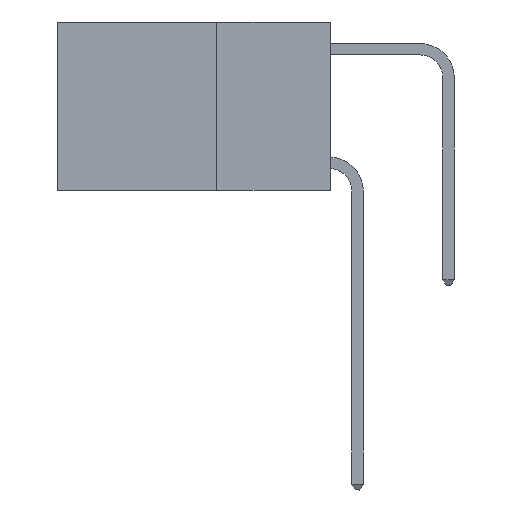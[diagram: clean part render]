
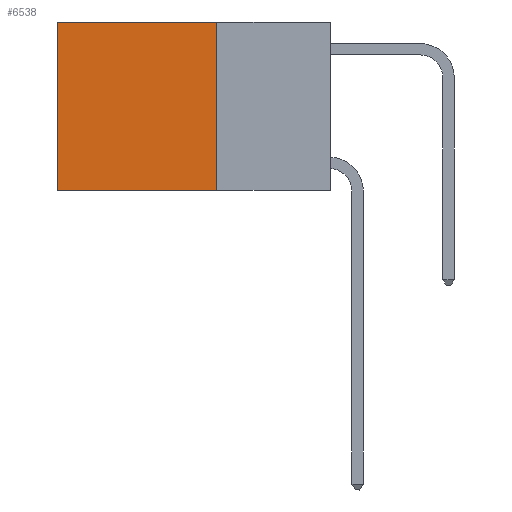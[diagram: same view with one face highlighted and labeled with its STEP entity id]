
A CAD part, left-side view. The second image highlights one B-rep face of the part: STEP entity #6538.
In plain terms, the highlighted planar face has unit normal (-1, 0, 0).
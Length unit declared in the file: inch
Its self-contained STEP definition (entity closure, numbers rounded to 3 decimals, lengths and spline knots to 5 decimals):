
#830 = PLANE ( 'NONE',  #6631 ) ;
#2566 = EDGE_CURVE ( 'NONE', #31942, #11204, #31097, .T. ) ;
#3371 = DIRECTION ( 'NONE',  ( 0., 0., -1. ) ) ;
#3516 = FACE_OUTER_BOUND ( 'NONE', #16178, .T. ) ;
#3772 = ORIENTED_EDGE ( 'NONE', *, *, #16917, .F. ) ;
#5088 = VECTOR ( 'NONE', #30983, 39.37008 ) ;
#5108 = CARTESIAN_POINT ( 'NONE',  ( 0.2625, 0.25, -0.37 ) ) ;
#5208 = CARTESIAN_POINT ( 'NONE',  ( 0.2625, 0.6, 0. ) ) ;
#5916 = LINE ( 'NONE', #5108, #5088 ) ;
#6202 = LINE ( 'NONE', #27113, #25265 ) ;
#6538 = ADVANCED_FACE ( 'NONE', ( #3516 ), #830, .F. ) ;
#6631 = AXIS2_PLACEMENT_3D ( 'NONE', #16211, #18812, #3371 ) ;
#7097 = CARTESIAN_POINT ( 'NONE',  ( 0.2625, 0.6, 0. ) ) ;
#8294 = EDGE_CURVE ( 'NONE', #31942, #12168, #6202, .T. ) ;
#8778 = CARTESIAN_POINT ( 'NONE',  ( 0.2625, 0.25, -0.37 ) ) ;
#8944 = DIRECTION ( 'NONE',  ( 0., 0., -1. ) ) ;
#9785 = EDGE_CURVE ( 'NONE', #11204, #24793, #14121, .T. ) ;
#10416 = VECTOR ( 'NONE', #23426, 39.37008 ) ;
#11204 = VERTEX_POINT ( 'NONE', #5208 ) ;
#11649 = VECTOR ( 'NONE', #27842, 39.37008 ) ;
#12168 = VERTEX_POINT ( 'NONE', #8778 ) ;
#12900 = CARTESIAN_POINT ( 'NONE',  ( 0.2625, 0.25, 0. ) ) ;
#14121 = LINE ( 'NONE', #7097, #11649 ) ;
#16178 = EDGE_LOOP ( 'NONE', ( #24566, #3772, #21248, #17769 ) ) ;
#16211 = CARTESIAN_POINT ( 'NONE',  ( 0.2625, 0.25, 0. ) ) ;
#16917 = EDGE_CURVE ( 'NONE', #12168, #24793, #5916, .T. ) ;
#17769 = ORIENTED_EDGE ( 'NONE', *, *, #2566, .T. ) ;
#18812 = DIRECTION ( 'NONE',  ( 1., 0., 0. ) ) ;
#19579 = CARTESIAN_POINT ( 'NONE',  ( 0.2625, 0.25, 0. ) ) ;
#21248 = ORIENTED_EDGE ( 'NONE', *, *, #8294, .F. ) ;
#23426 = DIRECTION ( 'NONE',  ( 0., 1., 0. ) ) ;
#24566 = ORIENTED_EDGE ( 'NONE', *, *, #9785, .T. ) ;
#24793 = VERTEX_POINT ( 'NONE', #33106 ) ;
#25265 = VECTOR ( 'NONE', #8944, 39.37008 ) ;
#27113 = CARTESIAN_POINT ( 'NONE',  ( 0.2625, 0.25, 0. ) ) ;
#27842 = DIRECTION ( 'NONE',  ( 0., 0., -1. ) ) ;
#30983 = DIRECTION ( 'NONE',  ( 0., 1., 0. ) ) ;
#31097 = LINE ( 'NONE', #12900, #10416 ) ;
#31942 = VERTEX_POINT ( 'NONE', #19579 ) ;
#33106 = CARTESIAN_POINT ( 'NONE',  ( 0.2625, 0.6, -0.37 ) ) ;
